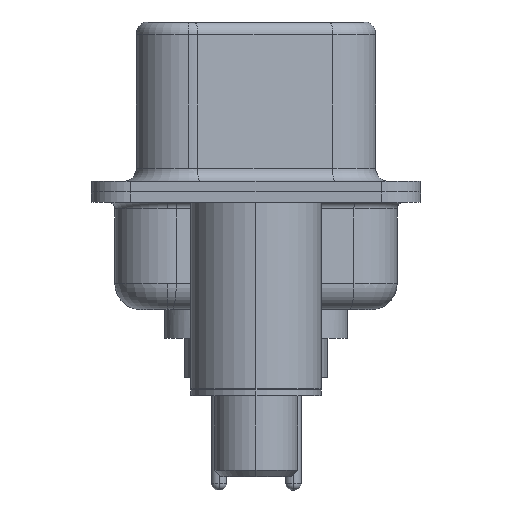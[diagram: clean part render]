
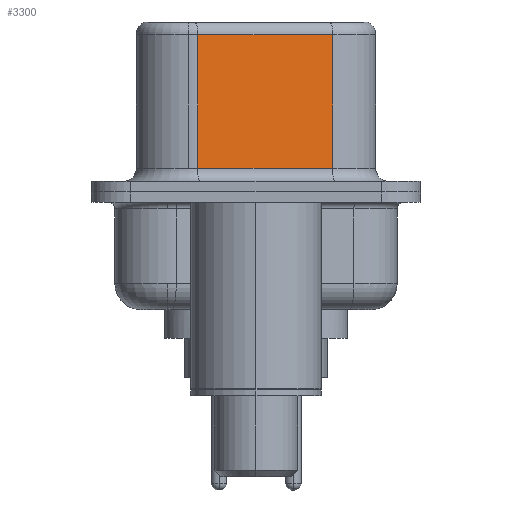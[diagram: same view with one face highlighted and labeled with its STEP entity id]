
A CAD part, left-side view. The second image highlights one B-rep face of the part: STEP entity #3300.
In plain terms, the highlighted planar face has unit normal (-0.985, -0.174, 0).
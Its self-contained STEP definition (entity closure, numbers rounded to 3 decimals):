
#1154 = ORIENTED_EDGE ( 'NONE', *, *, #18192, .T. ) ;
#2432 = VERTEX_POINT ( 'NONE', #8869 ) ;
#3300 = ADVANCED_FACE ( 'NONE', ( #13357 ), #4990, .F. ) ;
#3622 = VECTOR ( 'NONE', #15103, 1000. ) ;
#3896 = LINE ( 'NONE', #18538, #5011 ) ;
#4613 = CARTESIAN_POINT ( 'NONE',  ( 3.675, 2.233, 6.52 ) ) ;
#4990 = PLANE ( 'NONE',  #21955 ) ;
#5011 = VECTOR ( 'NONE', #6391, 1000. ) ;
#5327 = CARTESIAN_POINT ( 'NONE',  ( 4.585, -2.927, 6.52 ) ) ;
#5329 = EDGE_CURVE ( 'NONE', #7196, #2432, #20868, .T. ) ;
#6391 = DIRECTION ( 'NONE',  ( 0., 0., -1. ) ) ;
#6550 = ORIENTED_EDGE ( 'NONE', *, *, #7956, .T. ) ;
#7148 = CARTESIAN_POINT ( 'NONE',  ( 4.585, -2.927, 0.9 ) ) ;
#7196 = VERTEX_POINT ( 'NONE', #9754 ) ;
#7956 = EDGE_CURVE ( 'NONE', #2432, #14620, #8294, .T. ) ;
#8294 = LINE ( 'NONE', #4613, #3622 ) ;
#8869 = CARTESIAN_POINT ( 'NONE',  ( 3.675, 2.233, 6.02 ) ) ;
#9158 = EDGE_CURVE ( 'NONE', #7196, #21438, #3896, .T. ) ;
#9448 = DIRECTION ( 'NONE',  ( -0.174, 0.985, 0. ) ) ;
#9754 = CARTESIAN_POINT ( 'NONE',  ( 4.585, -2.927, 6.02 ) ) ;
#10351 = CARTESIAN_POINT ( 'NONE',  ( 3.675, 2.233, 0.9 ) ) ;
#10693 = DIRECTION ( 'NONE',  ( 0.174, -0.985, 0. ) ) ;
#12216 = VECTOR ( 'NONE', #9448, 1000. ) ;
#12316 = LINE ( 'NONE', #7148, #20976 ) ;
#12795 = ORIENTED_EDGE ( 'NONE', *, *, #5329, .T. ) ;
#13357 = FACE_OUTER_BOUND ( 'NONE', #19201, .T. ) ;
#13449 = CARTESIAN_POINT ( 'NONE',  ( 4.585, -2.927, 6.02 ) ) ;
#14620 = VERTEX_POINT ( 'NONE', #10351 ) ;
#15103 = DIRECTION ( 'NONE',  ( 0., 0., -1. ) ) ;
#17447 = CARTESIAN_POINT ( 'NONE',  ( 4.585, -2.927, 0.9 ) ) ;
#18192 = EDGE_CURVE ( 'NONE', #14620, #21438, #12316, .T. ) ;
#18538 = CARTESIAN_POINT ( 'NONE',  ( 4.585, -2.927, 6.52 ) ) ;
#19201 = EDGE_LOOP ( 'NONE', ( #19249, #12795, #6550, #1154 ) ) ;
#19249 = ORIENTED_EDGE ( 'NONE', *, *, #9158, .F. ) ;
#20868 = LINE ( 'NONE', #13449, #12216 ) ;
#20976 = VECTOR ( 'NONE', #10693, 1000. ) ;
#21438 = VERTEX_POINT ( 'NONE', #17447 ) ;
#21515 = DIRECTION ( 'NONE',  ( 0.985, 0.174, 0. ) ) ;
#21580 = DIRECTION ( 'NONE',  ( -0.174, 0.985, 0. ) ) ;
#21955 = AXIS2_PLACEMENT_3D ( 'NONE', #5327, #21515, #21580 ) ;
